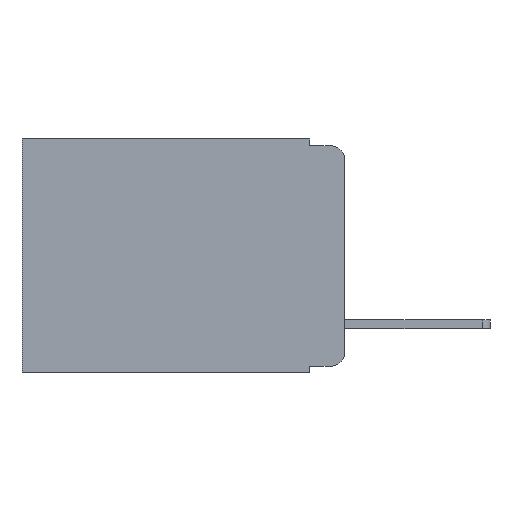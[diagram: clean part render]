
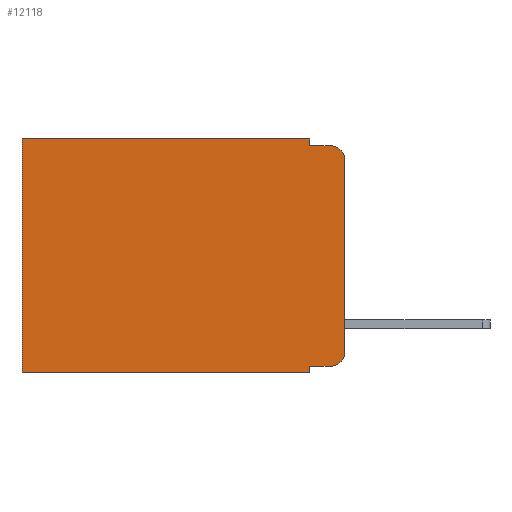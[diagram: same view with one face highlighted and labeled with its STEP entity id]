
A CAD part, left-side view. The second image highlights one B-rep face of the part: STEP entity #12118.
In plain terms, the highlighted planar face has unit normal (-1, 0, 0).
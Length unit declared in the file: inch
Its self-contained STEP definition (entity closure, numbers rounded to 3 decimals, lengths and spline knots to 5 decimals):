
#26 = DIRECTION ( 'NONE',  ( 0., 0., -1. ) ) ;
#154 = EDGE_CURVE ( 'NONE', #13719, #8048, #7636, .T. ) ;
#256 = CIRCLE ( 'NONE', #7328, 0.02 ) ;
#314 = DIRECTION ( 'NONE',  ( 0., 0., -1. ) ) ;
#1028 = VECTOR ( 'NONE', #5740, 39.37008 ) ;
#1101 = LINE ( 'NONE', #3368, #10599 ) ;
#1257 = CARTESIAN_POINT ( 'NONE',  ( 0.298, 0., 0. ) ) ;
#1770 = EDGE_CURVE ( 'NONE', #3129, #7947, #8765, .T. ) ;
#1806 = DIRECTION ( 'NONE',  ( 0., 1., 0. ) ) ;
#1851 = EDGE_CURVE ( 'NONE', #7947, #3935, #4278, .T. ) ;
#2002 = CARTESIAN_POINT ( 'NONE',  ( 0.298, 0.051, -0.01 ) ) ;
#2181 = VECTOR ( 'NONE', #1806, 39.37008 ) ;
#2675 = CARTESIAN_POINT ( 'NONE',  ( 0.298, 0.051, 0. ) ) ;
#2767 = VECTOR ( 'NONE', #4515, 39.37008 ) ;
#2852 = VECTOR ( 'NONE', #9452, 39.37008 ) ;
#3084 = DIRECTION ( 'NONE',  ( -1., 0., 0. ) ) ;
#3129 = VERTEX_POINT ( 'NONE', #14517 ) ;
#3368 = CARTESIAN_POINT ( 'NONE',  ( 0.298, 0., -0.343 ) ) ;
#3475 = ORIENTED_EDGE ( 'NONE', *, *, #5132, .F. ) ;
#3935 = VERTEX_POINT ( 'NONE', #11894 ) ;
#3956 = ORIENTED_EDGE ( 'NONE', *, *, #1851, .T. ) ;
#4158 = ORIENTED_EDGE ( 'NONE', *, *, #1770, .T. ) ;
#4278 = LINE ( 'NONE', #11731, #1028 ) ;
#4299 = EDGE_CURVE ( 'NONE', #3129, #5683, #4793, .T. ) ;
#4515 = DIRECTION ( 'NONE',  ( 0., -1., 0. ) ) ;
#4793 = LINE ( 'NONE', #15634, #14115 ) ;
#4934 = CARTESIAN_POINT ( 'NONE',  ( 0.298, 0.051, -0.343 ) ) ;
#5132 = EDGE_CURVE ( 'NONE', #5683, #11673, #9488, .T. ) ;
#5217 = DIRECTION ( 'NONE',  ( 0., 0., -1. ) ) ;
#5683 = VERTEX_POINT ( 'NONE', #6753 ) ;
#5740 = DIRECTION ( 'NONE',  ( 0., 0., -1. ) ) ;
#6753 = CARTESIAN_POINT ( 'NONE',  ( 0.298, 0.051, -0.01 ) ) ;
#6818 = EDGE_CURVE ( 'NONE', #12732, #11673, #256, .T. ) ;
#7122 = FACE_OUTER_BOUND ( 'NONE', #7855, .T. ) ;
#7328 = AXIS2_PLACEMENT_3D ( 'NONE', #14896, #7714, #314 ) ;
#7434 = DIRECTION ( 'NONE',  ( 1., 0., 0. ) ) ;
#7636 = LINE ( 'NONE', #2675, #13706 ) ;
#7714 = DIRECTION ( 'NONE',  ( -1., 0., 0. ) ) ;
#7855 = EDGE_LOOP ( 'NONE', ( #11374, #12613, #3475, #10470, #4158, #3956, #11278, #11598, #9649, #11722 ) ) ;
#7947 = VERTEX_POINT ( 'NONE', #8531 ) ;
#8048 = VERTEX_POINT ( 'NONE', #4934 ) ;
#8374 = CARTESIAN_POINT ( 'NONE',  ( 0.298, 0., 0. ) ) ;
#8531 = CARTESIAN_POINT ( 'NONE',  ( 0.298, 0.473, 0. ) ) ;
#8765 = LINE ( 'NONE', #8374, #2181 ) ;
#9142 = CARTESIAN_POINT ( 'NONE',  ( 0.298, 0.051, -0.333 ) ) ;
#9330 = LINE ( 'NONE', #15674, #12909 ) ;
#9333 = EDGE_CURVE ( 'NONE', #12732, #12571, #9330, .T. ) ;
#9452 = DIRECTION ( 'NONE',  ( 0., -1., 0. ) ) ;
#9488 = LINE ( 'NONE', #2002, #2852 ) ;
#9649 = ORIENTED_EDGE ( 'NONE', *, *, #15133, .T. ) ;
#9879 = DIRECTION ( 'NONE',  ( 0., 0., -1. ) ) ;
#10070 = CARTESIAN_POINT ( 'NONE',  ( 0.298, 0., -0.03 ) ) ;
#10470 = ORIENTED_EDGE ( 'NONE', *, *, #4299, .F. ) ;
#10526 = CARTESIAN_POINT ( 'NONE',  ( 0.298, 0.02, -0.313 ) ) ;
#10599 = VECTOR ( 'NONE', #10812, 39.37008 ) ;
#10772 = CIRCLE ( 'NONE', #15229, 0.02 ) ;
#10812 = DIRECTION ( 'NONE',  ( 0., 1., 0. ) ) ;
#10927 = CARTESIAN_POINT ( 'NONE',  ( 0.298, 0., -0.313 ) ) ;
#11278 = ORIENTED_EDGE ( 'NONE', *, *, #13065, .F. ) ;
#11374 = ORIENTED_EDGE ( 'NONE', *, *, #9333, .F. ) ;
#11598 = ORIENTED_EDGE ( 'NONE', *, *, #154, .F. ) ;
#11664 = AXIS2_PLACEMENT_3D ( 'NONE', #1257, #7434, #26 ) ;
#11673 = VERTEX_POINT ( 'NONE', #12587 ) ;
#11722 = ORIENTED_EDGE ( 'NONE', *, *, #14383, .T. ) ;
#11731 = CARTESIAN_POINT ( 'NONE',  ( 0.298, 0.473, 0. ) ) ;
#11747 = DIRECTION ( 'NONE',  ( 0., 0., -1. ) ) ;
#11894 = CARTESIAN_POINT ( 'NONE',  ( 0.298, 0.473, -0.343 ) ) ;
#12118 = ADVANCED_FACE ( 'NONE', ( #7122 ), #14648, .F. ) ;
#12571 = VERTEX_POINT ( 'NONE', #10927 ) ;
#12587 = CARTESIAN_POINT ( 'NONE',  ( 0.298, 0.02, -0.01 ) ) ;
#12613 = ORIENTED_EDGE ( 'NONE', *, *, #6818, .T. ) ;
#12732 = VERTEX_POINT ( 'NONE', #10070 ) ;
#12909 = VECTOR ( 'NONE', #9879, 39.37008 ) ;
#13065 = EDGE_CURVE ( 'NONE', #8048, #3935, #1101, .T. ) ;
#13105 = CARTESIAN_POINT ( 'NONE',  ( 0.298, 0.051, -0.333 ) ) ;
#13706 = VECTOR ( 'NONE', #5217, 39.37008 ) ;
#13719 = VERTEX_POINT ( 'NONE', #9142 ) ;
#13773 = CARTESIAN_POINT ( 'NONE',  ( 0.298, 0.02, -0.333 ) ) ;
#14115 = VECTOR ( 'NONE', #14668, 39.37008 ) ;
#14282 = VERTEX_POINT ( 'NONE', #13773 ) ;
#14383 = EDGE_CURVE ( 'NONE', #14282, #12571, #10772, .T. ) ;
#14517 = CARTESIAN_POINT ( 'NONE',  ( 0.298, 0.051, 0. ) ) ;
#14648 = PLANE ( 'NONE',  #11664 ) ;
#14668 = DIRECTION ( 'NONE',  ( 0., 0., -1. ) ) ;
#14896 = CARTESIAN_POINT ( 'NONE',  ( 0.298, 0.02, -0.03 ) ) ;
#15133 = EDGE_CURVE ( 'NONE', #13719, #14282, #15611, .T. ) ;
#15229 = AXIS2_PLACEMENT_3D ( 'NONE', #10526, #3084, #11747 ) ;
#15611 = LINE ( 'NONE', #13105, #2767 ) ;
#15634 = CARTESIAN_POINT ( 'NONE',  ( 0.298, 0.051, 0. ) ) ;
#15674 = CARTESIAN_POINT ( 'NONE',  ( 0.298, 0., 0. ) ) ;
